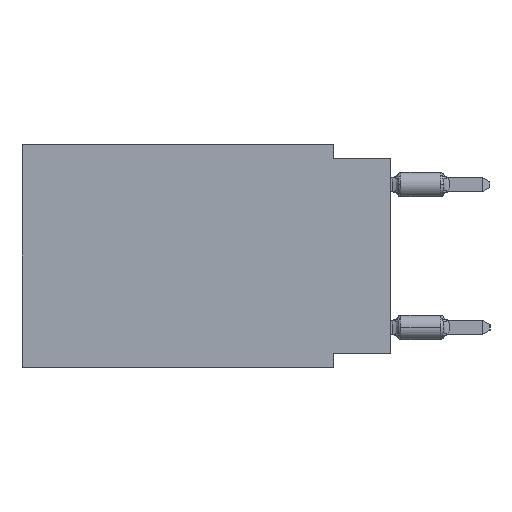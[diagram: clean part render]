
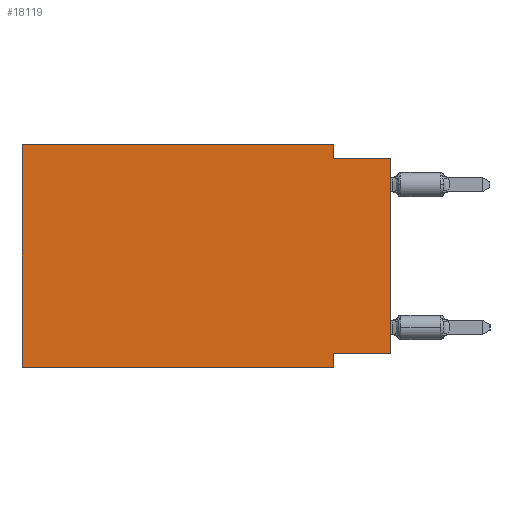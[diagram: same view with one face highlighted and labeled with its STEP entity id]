
A CAD part, left-side view. The second image highlights one B-rep face of the part: STEP entity #18119.
In plain terms, the highlighted planar face has unit normal (-1, 0, 0).
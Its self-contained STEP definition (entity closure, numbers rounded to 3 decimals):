
#86 = DIRECTION ( 'NONE',  ( 0., 0., -1. ) ) ;
#3744 = ORIENTED_EDGE ( 'NONE', *, *, #49222, .F. ) ;
#3989 = ORIENTED_EDGE ( 'NONE', *, *, #62299, .F. ) ;
#5408 = LINE ( 'NONE', #26151, #57064 ) ;
#5851 = CARTESIAN_POINT ( 'NONE',  ( 0., 0., -0.635 ) ) ;
#6287 = CARTESIAN_POINT ( 'NONE',  ( 0., 16.383, 0. ) ) ;
#6792 = VECTOR ( 'NONE', #9821, 1000. ) ;
#6972 = DIRECTION ( 'NONE',  ( 0., 0., -1. ) ) ;
#8607 = VERTEX_POINT ( 'NONE', #64791 ) ;
#9821 = DIRECTION ( 'NONE',  ( 0., -1., 0. ) ) ;
#10941 = VERTEX_POINT ( 'NONE', #16038 ) ;
#12002 = EDGE_CURVE ( 'NONE', #10941, #59743, #24647, .T. ) ;
#12085 = ORIENTED_EDGE ( 'NONE', *, *, #16520, .F. ) ;
#14094 = VECTOR ( 'NONE', #20846, 1000. ) ;
#15169 = LINE ( 'NONE', #30909, #21262 ) ;
#16038 = CARTESIAN_POINT ( 'NONE',  ( 0., 0., -9.271 ) ) ;
#16520 = EDGE_CURVE ( 'NONE', #10941, #8607, #5408, .T. ) ;
#16609 = ORIENTED_EDGE ( 'NONE', *, *, #45371, .T. ) ;
#17407 = ORIENTED_EDGE ( 'NONE', *, *, #27676, .F. ) ;
#17441 = EDGE_LOOP ( 'NONE', ( #27811, #17407, #40374, #43401, #3744, #16609, #3989, #12085 ) ) ;
#18110 = VERTEX_POINT ( 'NONE', #48872 ) ;
#18119 = ADVANCED_FACE ( 'NONE', ( #39170 ), #39827, .F. ) ;
#19850 = CARTESIAN_POINT ( 'NONE',  ( 0., 16.383, 0. ) ) ;
#20692 = CARTESIAN_POINT ( 'NONE',  ( 0., 2.54, -9.906 ) ) ;
#20846 = DIRECTION ( 'NONE',  ( 0., -1., 0. ) ) ;
#21257 = CARTESIAN_POINT ( 'NONE',  ( 0., 2.54, -0.635 ) ) ;
#21262 = VECTOR ( 'NONE', #86, 1000. ) ;
#22040 = CARTESIAN_POINT ( 'NONE',  ( 0., 2.54, 0. ) ) ;
#23878 = LINE ( 'NONE', #63434, #49021 ) ;
#24141 = LINE ( 'NONE', #28173, #64699 ) ;
#24647 = LINE ( 'NONE', #42847, #60997 ) ;
#26151 = CARTESIAN_POINT ( 'NONE',  ( 0., 0., -9.271 ) ) ;
#27676 = EDGE_CURVE ( 'NONE', #60977, #59743, #40950, .T. ) ;
#27811 = ORIENTED_EDGE ( 'NONE', *, *, #12002, .T. ) ;
#28173 = CARTESIAN_POINT ( 'NONE',  ( 0., 16.383, 0. ) ) ;
#29872 = VERTEX_POINT ( 'NONE', #6287 ) ;
#30909 = CARTESIAN_POINT ( 'NONE',  ( 0., 2.54, -9.906 ) ) ;
#36166 = EDGE_CURVE ( 'NONE', #29872, #18110, #65747, .T. ) ;
#36893 = AXIS2_PLACEMENT_3D ( 'NONE', #50222, #60262, #43843 ) ;
#38531 = VERTEX_POINT ( 'NONE', #20692 ) ;
#38963 = DIRECTION ( 'NONE',  ( 0., -1., 0. ) ) ;
#39170 = FACE_OUTER_BOUND ( 'NONE', #17441, .T. ) ;
#39827 = PLANE ( 'NONE',  #36893 ) ;
#40058 = EDGE_CURVE ( 'NONE', #18110, #60977, #52843, .T. ) ;
#40374 = ORIENTED_EDGE ( 'NONE', *, *, #40058, .F. ) ;
#40950 = LINE ( 'NONE', #61400, #14094 ) ;
#42847 = CARTESIAN_POINT ( 'NONE',  ( 0., 0., 0. ) ) ;
#43401 = ORIENTED_EDGE ( 'NONE', *, *, #36166, .F. ) ;
#43843 = DIRECTION ( 'NONE',  ( 0., 0., -1. ) ) ;
#45075 = DIRECTION ( 'NONE',  ( 0., 0., 1. ) ) ;
#45371 = EDGE_CURVE ( 'NONE', #65793, #38531, #23878, .T. ) ;
#48872 = CARTESIAN_POINT ( 'NONE',  ( 0., 2.54, 0. ) ) ;
#49021 = VECTOR ( 'NONE', #38963, 1000. ) ;
#49222 = EDGE_CURVE ( 'NONE', #65793, #29872, #24141, .T. ) ;
#50222 = CARTESIAN_POINT ( 'NONE',  ( 0., 16.383, 0. ) ) ;
#52843 = LINE ( 'NONE', #22040, #59416 ) ;
#57064 = VECTOR ( 'NONE', #61351, 1000. ) ;
#58661 = DIRECTION ( 'NONE',  ( 0., 0., 1. ) ) ;
#58882 = CARTESIAN_POINT ( 'NONE',  ( 0., 16.383, -9.906 ) ) ;
#59416 = VECTOR ( 'NONE', #6972, 1000. ) ;
#59743 = VERTEX_POINT ( 'NONE', #5851 ) ;
#60262 = DIRECTION ( 'NONE',  ( 1., 0., 0. ) ) ;
#60977 = VERTEX_POINT ( 'NONE', #21257 ) ;
#60997 = VECTOR ( 'NONE', #45075, 1000. ) ;
#61351 = DIRECTION ( 'NONE',  ( 0., 1., 0. ) ) ;
#61400 = CARTESIAN_POINT ( 'NONE',  ( 0., 0., -0.635 ) ) ;
#62299 = EDGE_CURVE ( 'NONE', #8607, #38531, #15169, .T. ) ;
#63434 = CARTESIAN_POINT ( 'NONE',  ( 0., 16.383, -9.906 ) ) ;
#64699 = VECTOR ( 'NONE', #58661, 1000. ) ;
#64791 = CARTESIAN_POINT ( 'NONE',  ( 0., 2.54, -9.271 ) ) ;
#65747 = LINE ( 'NONE', #19850, #6792 ) ;
#65793 = VERTEX_POINT ( 'NONE', #58882 ) ;
